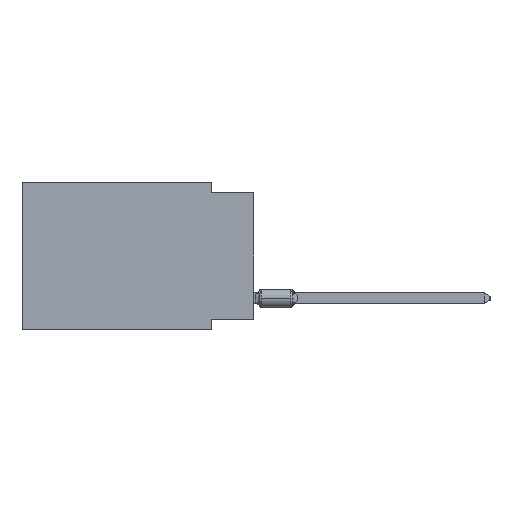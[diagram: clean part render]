
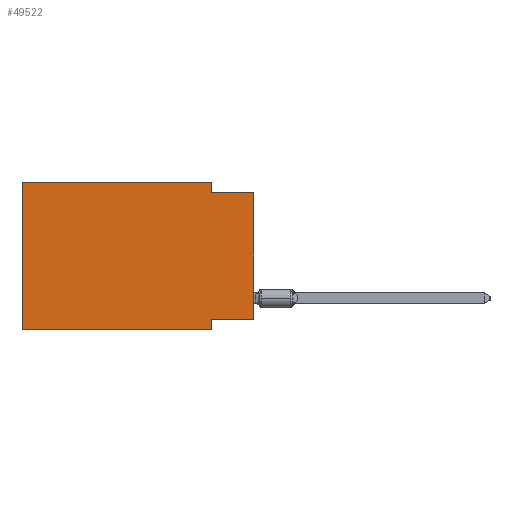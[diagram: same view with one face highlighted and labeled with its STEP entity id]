
A CAD part, left-side view. The second image highlights one B-rep face of the part: STEP entity #49522.
In plain terms, the highlighted planar face has unit normal (-1, 0, 0).
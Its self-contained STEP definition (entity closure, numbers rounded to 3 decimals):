
#522 = CARTESIAN_POINT ( 'NONE',  ( 0., 2.54, -8.255 ) ) ;
#739 = VERTEX_POINT ( 'NONE', #522 ) ;
#773 = ORIENTED_EDGE ( 'NONE', *, *, #48425, .T. ) ;
#1055 = DIRECTION ( 'NONE',  ( 0., -1., 0. ) ) ;
#1457 = EDGE_CURVE ( 'NONE', #739, #35299, #5064, .T. ) ;
#1824 = EDGE_CURVE ( 'NONE', #46859, #50076, #52016, .T. ) ;
#3034 = CARTESIAN_POINT ( 'NONE',  ( 0., 2.54, 0. ) ) ;
#3638 = CARTESIAN_POINT ( 'NONE',  ( 0., 13.97, 0. ) ) ;
#3765 = VECTOR ( 'NONE', #10775, 1000. ) ;
#4970 = PLANE ( 'NONE',  #15763 ) ;
#5064 = LINE ( 'NONE', #46832, #5330 ) ;
#5330 = VECTOR ( 'NONE', #8239, 1000. ) ;
#7297 = DIRECTION ( 'NONE',  ( 0., -1., 0. ) ) ;
#8067 = ORIENTED_EDGE ( 'NONE', *, *, #21620, .F. ) ;
#8239 = DIRECTION ( 'NONE',  ( 0., 0., -1. ) ) ;
#10360 = ORIENTED_EDGE ( 'NONE', *, *, #15729, .F. ) ;
#10710 = ORIENTED_EDGE ( 'NONE', *, *, #37168, .F. ) ;
#10775 = DIRECTION ( 'NONE',  ( 0., 0., 1. ) ) ;
#11184 = DIRECTION ( 'NONE',  ( 0., 0., -1. ) ) ;
#11525 = CARTESIAN_POINT ( 'NONE',  ( 0., 0., -0.635 ) ) ;
#12058 = VECTOR ( 'NONE', #7297, 1000. ) ;
#13157 = CARTESIAN_POINT ( 'NONE',  ( 0., 0., -0.635 ) ) ;
#13680 = DIRECTION ( 'NONE',  ( 0., -1., 0. ) ) ;
#14026 = CARTESIAN_POINT ( 'NONE',  ( 0., 13.97, -8.89 ) ) ;
#14583 = EDGE_CURVE ( 'NONE', #20890, #739, #18417, .T. ) ;
#14979 = DIRECTION ( 'NONE',  ( 0., 0., 1. ) ) ;
#15729 = EDGE_CURVE ( 'NONE', #40860, #31613, #32463, .T. ) ;
#15763 = AXIS2_PLACEMENT_3D ( 'NONE', #51727, #26068, #47758 ) ;
#16491 = EDGE_CURVE ( 'NONE', #40860, #35299, #19310, .T. ) ;
#17855 = CARTESIAN_POINT ( 'NONE',  ( 0., 2.54, -0.635 ) ) ;
#17925 = VECTOR ( 'NONE', #1055, 1000. ) ;
#18417 = LINE ( 'NONE', #47995, #20994 ) ;
#19310 = LINE ( 'NONE', #36506, #43584 ) ;
#20890 = VERTEX_POINT ( 'NONE', #26476 ) ;
#20994 = VECTOR ( 'NONE', #39266, 1000. ) ;
#21564 = FACE_OUTER_BOUND ( 'NONE', #29746, .T. ) ;
#21620 = EDGE_CURVE ( 'NONE', #22048, #46859, #46383, .T. ) ;
#22048 = VERTEX_POINT ( 'NONE', #41810 ) ;
#26068 = DIRECTION ( 'NONE',  ( 1., 0., 0. ) ) ;
#26152 = ORIENTED_EDGE ( 'NONE', *, *, #16491, .T. ) ;
#26476 = CARTESIAN_POINT ( 'NONE',  ( 0., 0., -8.255 ) ) ;
#29174 = VECTOR ( 'NONE', #14979, 1000. ) ;
#29355 = ORIENTED_EDGE ( 'NONE', *, *, #1824, .F. ) ;
#29746 = EDGE_LOOP ( 'NONE', ( #773, #29355, #8067, #10710, #10360, #26152, #51814, #40498 ) ) ;
#31613 = VERTEX_POINT ( 'NONE', #50222 ) ;
#32463 = LINE ( 'NONE', #36419, #3765 ) ;
#35299 = VERTEX_POINT ( 'NONE', #37405 ) ;
#36419 = CARTESIAN_POINT ( 'NONE',  ( 0., 13.97, 0. ) ) ;
#36506 = CARTESIAN_POINT ( 'NONE',  ( 0., 13.97, -8.89 ) ) ;
#37168 = EDGE_CURVE ( 'NONE', #31613, #22048, #41098, .T. ) ;
#37405 = CARTESIAN_POINT ( 'NONE',  ( 0., 2.54, -8.89 ) ) ;
#39266 = DIRECTION ( 'NONE',  ( 0., 1., 0. ) ) ;
#40498 = ORIENTED_EDGE ( 'NONE', *, *, #14583, .F. ) ;
#40860 = VERTEX_POINT ( 'NONE', #14026 ) ;
#41098 = LINE ( 'NONE', #3638, #12058 ) ;
#41799 = VECTOR ( 'NONE', #11184, 1000. ) ;
#41810 = CARTESIAN_POINT ( 'NONE',  ( 0., 2.54, 0. ) ) ;
#43584 = VECTOR ( 'NONE', #13680, 1000. ) ;
#45412 = LINE ( 'NONE', #53864, #29174 ) ;
#46383 = LINE ( 'NONE', #3034, #41799 ) ;
#46832 = CARTESIAN_POINT ( 'NONE',  ( 0., 2.54, -8.89 ) ) ;
#46859 = VERTEX_POINT ( 'NONE', #17855 ) ;
#47758 = DIRECTION ( 'NONE',  ( 0., 0., -1. ) ) ;
#47995 = CARTESIAN_POINT ( 'NONE',  ( 0., 0., -8.255 ) ) ;
#48425 = EDGE_CURVE ( 'NONE', #20890, #50076, #45412, .T. ) ;
#49522 = ADVANCED_FACE ( 'NONE', ( #21564 ), #4970, .F. ) ;
#50076 = VERTEX_POINT ( 'NONE', #11525 ) ;
#50222 = CARTESIAN_POINT ( 'NONE',  ( 0., 13.97, 0. ) ) ;
#51727 = CARTESIAN_POINT ( 'NONE',  ( 0., 13.97, 0. ) ) ;
#51814 = ORIENTED_EDGE ( 'NONE', *, *, #1457, .F. ) ;
#52016 = LINE ( 'NONE', #13157, #17925 ) ;
#53864 = CARTESIAN_POINT ( 'NONE',  ( 0., 0., 0. ) ) ;
